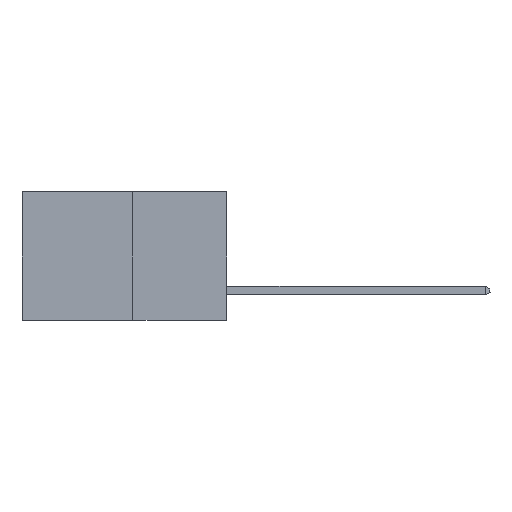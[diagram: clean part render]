
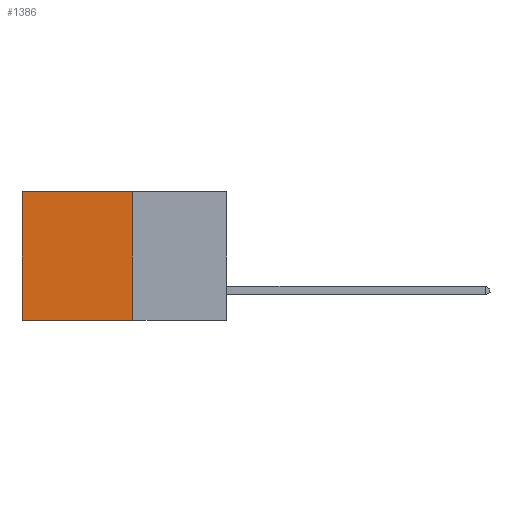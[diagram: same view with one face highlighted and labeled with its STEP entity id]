
A CAD part, left-side view. The second image highlights one B-rep face of the part: STEP entity #1386.
In plain terms, the highlighted planar face has unit normal (-1, 0, 0).
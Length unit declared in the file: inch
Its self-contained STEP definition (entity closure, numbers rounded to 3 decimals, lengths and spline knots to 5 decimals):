
#617 = CARTESIAN_POINT ( 'NONE',  ( 0.277, 0.59, -0.37 ) ) ;
#1386 = ADVANCED_FACE ( 'NONE', ( #27817 ), #3339, .F. ) ;
#1824 = CARTESIAN_POINT ( 'NONE',  ( 0.277, 0.59, 0. ) ) ;
#1869 = DIRECTION ( 'NONE',  ( 0., 0., -1. ) ) ;
#2506 = VECTOR ( 'NONE', #24339, 39.37008 ) ;
#3339 = PLANE ( 'NONE',  #25269 ) ;
#5852 = EDGE_CURVE ( 'NONE', #28665, #24843, #23294, .T. ) ;
#6213 = VERTEX_POINT ( 'NONE', #10311 ) ;
#6551 = ORIENTED_EDGE ( 'NONE', *, *, #18670, .T. ) ;
#9019 = CARTESIAN_POINT ( 'NONE',  ( 0.277, 0.27, -0.37 ) ) ;
#10311 = CARTESIAN_POINT ( 'NONE',  ( 0.277, 0.27, -0.37 ) ) ;
#11132 = LINE ( 'NONE', #13219, #29040 ) ;
#11286 = ORIENTED_EDGE ( 'NONE', *, *, #12369, .F. ) ;
#11838 = EDGE_CURVE ( 'NONE', #6213, #24843, #26529, .T. ) ;
#12369 = EDGE_CURVE ( 'NONE', #23719, #6213, #11132, .T. ) ;
#12588 = CARTESIAN_POINT ( 'NONE',  ( 0.277, 0.27, 0. ) ) ;
#13219 = CARTESIAN_POINT ( 'NONE',  ( 0.277, 0.27, -0.37 ) ) ;
#14104 = VECTOR ( 'NONE', #25419, 39.37008 ) ;
#15555 = CARTESIAN_POINT ( 'NONE',  ( 0.277, 0.27, 0. ) ) ;
#16509 = LINE ( 'NONE', #12588, #2506 ) ;
#18670 = EDGE_CURVE ( 'NONE', #23719, #28665, #16509, .T. ) ;
#18766 = ORIENTED_EDGE ( 'NONE', *, *, #11838, .F. ) ;
#19945 = DIRECTION ( 'NONE',  ( 0., 0., -1. ) ) ;
#20994 = DIRECTION ( 'NONE',  ( 1., 0., 0. ) ) ;
#22058 = CARTESIAN_POINT ( 'NONE',  ( 0.277, 0.27, -0.37 ) ) ;
#23030 = CARTESIAN_POINT ( 'NONE',  ( 0.277, 0.59, -0.37 ) ) ;
#23294 = LINE ( 'NONE', #23030, #28760 ) ;
#23719 = VERTEX_POINT ( 'NONE', #15555 ) ;
#24339 = DIRECTION ( 'NONE',  ( 0., 1., 0. ) ) ;
#24843 = VERTEX_POINT ( 'NONE', #617 ) ;
#24980 = DIRECTION ( 'NONE',  ( 0., 0., -1. ) ) ;
#25269 = AXIS2_PLACEMENT_3D ( 'NONE', #22058, #20994, #19945 ) ;
#25419 = DIRECTION ( 'NONE',  ( 0., 1., 0. ) ) ;
#26529 = LINE ( 'NONE', #9019, #14104 ) ;
#27541 = ORIENTED_EDGE ( 'NONE', *, *, #5852, .T. ) ;
#27817 = FACE_OUTER_BOUND ( 'NONE', #29776, .T. ) ;
#28665 = VERTEX_POINT ( 'NONE', #1824 ) ;
#28760 = VECTOR ( 'NONE', #1869, 39.37008 ) ;
#29040 = VECTOR ( 'NONE', #24980, 39.37008 ) ;
#29776 = EDGE_LOOP ( 'NONE', ( #27541, #18766, #11286, #6551 ) ) ;
